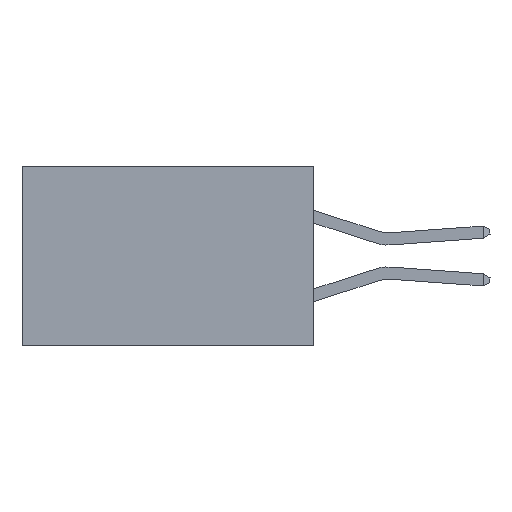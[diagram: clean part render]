
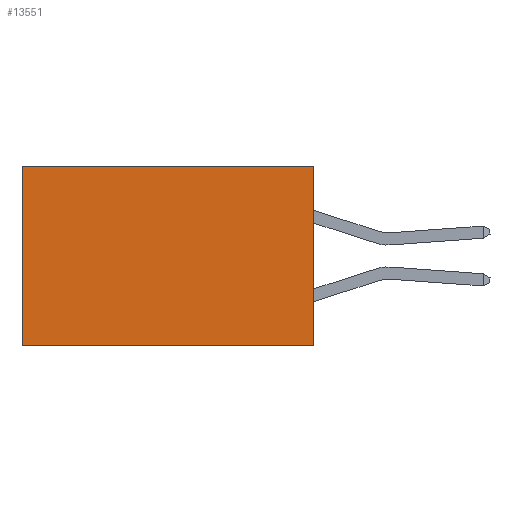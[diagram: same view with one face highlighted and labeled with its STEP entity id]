
A CAD part, left-side view. The second image highlights one B-rep face of the part: STEP entity #13551.
In plain terms, the highlighted planar face has unit normal (-1, 0, 0).
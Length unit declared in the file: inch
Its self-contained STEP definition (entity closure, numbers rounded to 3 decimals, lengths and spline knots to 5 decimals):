
#205 = CARTESIAN_POINT ( 'NONE',  ( 0.2875, 0., 0. ) ) ;
#683 = ORIENTED_EDGE ( 'NONE', *, *, #6354, .T. ) ;
#922 = CARTESIAN_POINT ( 'NONE',  ( 0.2875, 0., 0. ) ) ;
#1998 = ORIENTED_EDGE ( 'NONE', *, *, #27532, .F. ) ;
#2546 = PLANE ( 'NONE',  #28076 ) ;
#2897 = FACE_OUTER_BOUND ( 'NONE', #10373, .T. ) ;
#2965 = CARTESIAN_POINT ( 'NONE',  ( 0.2875, 0., -0.37 ) ) ;
#5491 = CARTESIAN_POINT ( 'NONE',  ( 0.2875, 0.6, 0. ) ) ;
#6354 = EDGE_CURVE ( 'NONE', #10846, #9275, #7823, .T. ) ;
#6611 = CARTESIAN_POINT ( 'NONE',  ( 0.2875, 0.6, 0. ) ) ;
#7079 = ORIENTED_EDGE ( 'NONE', *, *, #13774, .T. ) ;
#7764 = VERTEX_POINT ( 'NONE', #13101 ) ;
#7823 = LINE ( 'NONE', #5491, #19698 ) ;
#7926 = DIRECTION ( 'NONE',  ( 0., 0., -1. ) ) ;
#9275 = VERTEX_POINT ( 'NONE', #29511 ) ;
#9483 = VERTEX_POINT ( 'NONE', #20783 ) ;
#10373 = EDGE_LOOP ( 'NONE', ( #683, #1998, #23794, #7079 ) ) ;
#10846 = VERTEX_POINT ( 'NONE', #6611 ) ;
#12301 = DIRECTION ( 'NONE',  ( 1., 0., 0. ) ) ;
#13101 = CARTESIAN_POINT ( 'NONE',  ( 0.2875, 0., 0. ) ) ;
#13551 = ADVANCED_FACE ( 'NONE', ( #2897 ), #2546, .F. ) ;
#13774 = EDGE_CURVE ( 'NONE', #7764, #10846, #23048, .T. ) ;
#15352 = DIRECTION ( 'NONE',  ( 0., 1., 0. ) ) ;
#16042 = VECTOR ( 'NONE', #15352, 39.37008 ) ;
#16844 = VECTOR ( 'NONE', #24146, 39.37008 ) ;
#19030 = VECTOR ( 'NONE', #26673, 39.37008 ) ;
#19698 = VECTOR ( 'NONE', #7926, 39.37008 ) ;
#19743 = EDGE_CURVE ( 'NONE', #7764, #9483, #29298, .T. ) ;
#20783 = CARTESIAN_POINT ( 'NONE',  ( 0.2875, 0., -0.37 ) ) ;
#23048 = LINE ( 'NONE', #922, #16042 ) ;
#23794 = ORIENTED_EDGE ( 'NONE', *, *, #19743, .F. ) ;
#24146 = DIRECTION ( 'NONE',  ( 0., 0., -1. ) ) ;
#25992 = LINE ( 'NONE', #2965, #19030 ) ;
#26361 = CARTESIAN_POINT ( 'NONE',  ( 0.2875, 0., 0. ) ) ;
#26673 = DIRECTION ( 'NONE',  ( 0., 1., 0. ) ) ;
#27532 = EDGE_CURVE ( 'NONE', #9483, #9275, #25992, .T. ) ;
#28076 = AXIS2_PLACEMENT_3D ( 'NONE', #26361, #12301, #28732 ) ;
#28732 = DIRECTION ( 'NONE',  ( 0., 0., -1. ) ) ;
#29298 = LINE ( 'NONE', #205, #16844 ) ;
#29511 = CARTESIAN_POINT ( 'NONE',  ( 0.2875, 0.6, -0.37 ) ) ;
